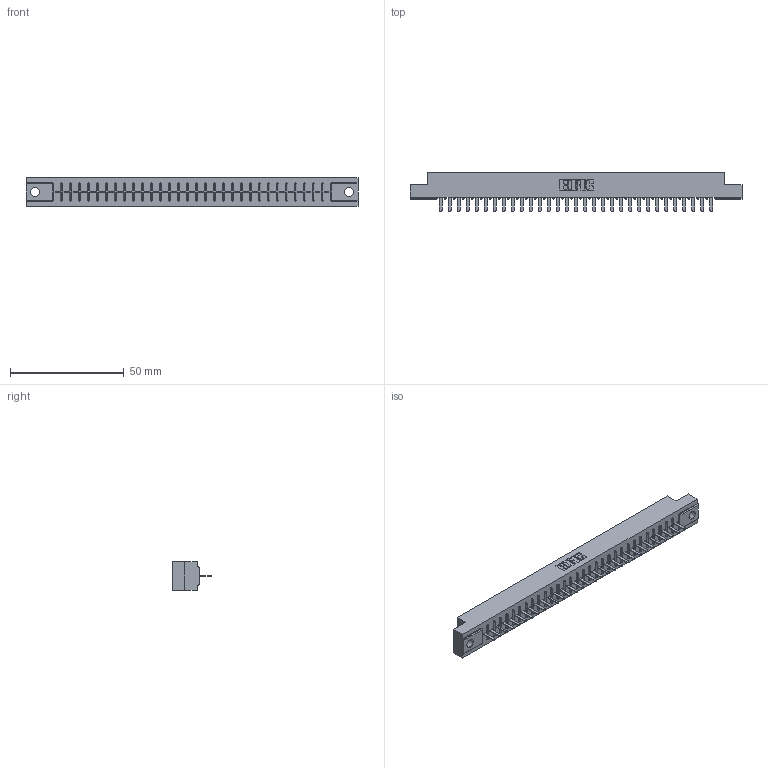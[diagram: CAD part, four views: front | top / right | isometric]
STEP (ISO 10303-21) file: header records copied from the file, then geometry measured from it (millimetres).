
FILE_DESCRIPTION (( 'STEP AP203' ), '1' );
FILE_NAME ('316-031-520-104.STEP', '2018-07-31T03:29:37', ( '' ), ( '' ), 'SwSTEP 2.0', 'SolidWorks 2016', '' );
FILE_SCHEMA (( 'CONFIG_CONTROL_DESIGN' ));
Length unit declared in the file: inch
Products named in the file (3): 306 Part_.156 Dia; 306-290-001_120; 316-031-520-104
Assembly tree (32 placements, depth 2):
  316-031-520-104
    306 Part_.156 Dia
    306-290-001_120  x31
Bounding box: 145.85 x 17.12 x 12.7 mm (x, y, z)
Volume: 15932.5 mm3; surface area: 16053.2 mm2
Topology: 32 solids, 32 shells, 2300 faces, 6459 edges, 4138 vertices
Faces by surface type: plane 1539, cylinder 637, sphere 124
Entity records: 30708 total; most frequent: CARTESIAN_POINT 5158, ORIENTED_EDGE 5110, DIRECTION 5079, EDGE_CURVE 2555, VECTOR 2001, LINE 2001, VERTEX_POINT 1618, AXIS2_PLACEMENT_3D 1539
